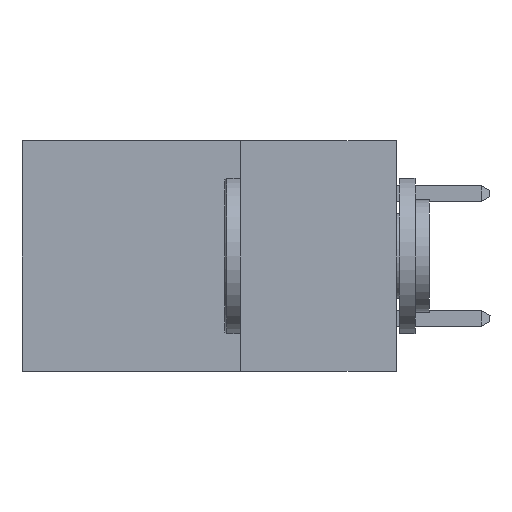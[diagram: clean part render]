
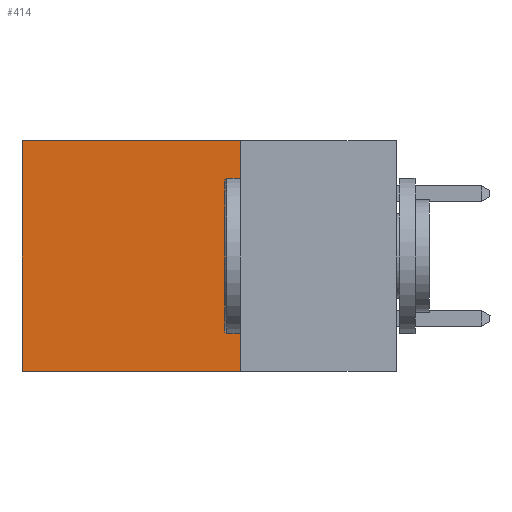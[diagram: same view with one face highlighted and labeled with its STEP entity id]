
A CAD part, left-side view. The second image highlights one B-rep face of the part: STEP entity #414.
In plain terms, the highlighted planar face has unit normal (-1, 0, 0).
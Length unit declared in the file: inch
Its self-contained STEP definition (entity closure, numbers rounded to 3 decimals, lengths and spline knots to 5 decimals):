
#123 = CARTESIAN_POINT ( 'NONE',  ( 0.2615, 0.6, -0.37 ) ) ;
#414 = ADVANCED_FACE ( 'NONE', ( #3703 ), #14101, .F. ) ;
#1155 = CARTESIAN_POINT ( 'NONE',  ( 0.2615, 0.6, 0. ) ) ;
#3271 = VECTOR ( 'NONE', #9508, 39.37008 ) ;
#3703 = FACE_OUTER_BOUND ( 'NONE', #8497, .T. ) ;
#3852 = VECTOR ( 'NONE', #13109, 39.37008 ) ;
#4131 = VERTEX_POINT ( 'NONE', #1155 ) ;
#4448 = VECTOR ( 'NONE', #7149, 39.37008 ) ;
#5177 = VERTEX_POINT ( 'NONE', #11991 ) ;
#6229 = VECTOR ( 'NONE', #7909, 39.37008 ) ;
#6248 = CARTESIAN_POINT ( 'NONE',  ( 0.2615, 0.25, -0.37 ) ) ;
#7024 = ORIENTED_EDGE ( 'NONE', *, *, #14370, .T. ) ;
#7149 = DIRECTION ( 'NONE',  ( 0., 1., 0. ) ) ;
#7431 = ORIENTED_EDGE ( 'NONE', *, *, #7670, .F. ) ;
#7547 = DIRECTION ( 'NONE',  ( 1., 0., 0. ) ) ;
#7670 = EDGE_CURVE ( 'NONE', #15599, #5177, #10167, .T. ) ;
#7909 = DIRECTION ( 'NONE',  ( 0., 0., -1. ) ) ;
#8202 = CARTESIAN_POINT ( 'NONE',  ( 0.2615, 0.25, -0.37 ) ) ;
#8461 = ORIENTED_EDGE ( 'NONE', *, *, #15417, .T. ) ;
#8497 = EDGE_LOOP ( 'NONE', ( #7024, #10496, #7431, #8461 ) ) ;
#9508 = DIRECTION ( 'NONE',  ( 0., 0., -1. ) ) ;
#10167 = LINE ( 'NONE', #8202, #3271 ) ;
#10496 = ORIENTED_EDGE ( 'NONE', *, *, #13069, .F. ) ;
#11783 = CARTESIAN_POINT ( 'NONE',  ( 0.2615, 0.25, -0.37 ) ) ;
#11800 = LINE ( 'NONE', #15019, #4448 ) ;
#11991 = CARTESIAN_POINT ( 'NONE',  ( 0.2615, 0.25, -0.37 ) ) ;
#13069 = EDGE_CURVE ( 'NONE', #5177, #16252, #14274, .T. ) ;
#13109 = DIRECTION ( 'NONE',  ( 0., 1., 0. ) ) ;
#13206 = LINE ( 'NONE', #123, #6229 ) ;
#14101 = PLANE ( 'NONE',  #14761 ) ;
#14274 = LINE ( 'NONE', #11783, #3852 ) ;
#14370 = EDGE_CURVE ( 'NONE', #4131, #16252, #13206, .T. ) ;
#14761 = AXIS2_PLACEMENT_3D ( 'NONE', #6248, #7547, #16730 ) ;
#15019 = CARTESIAN_POINT ( 'NONE',  ( 0.2615, 0.25, 0. ) ) ;
#15343 = CARTESIAN_POINT ( 'NONE',  ( 0.2615, 0.25, 0. ) ) ;
#15417 = EDGE_CURVE ( 'NONE', #15599, #4131, #11800, .T. ) ;
#15599 = VERTEX_POINT ( 'NONE', #15343 ) ;
#16099 = CARTESIAN_POINT ( 'NONE',  ( 0.2615, 0.6, -0.37 ) ) ;
#16252 = VERTEX_POINT ( 'NONE', #16099 ) ;
#16730 = DIRECTION ( 'NONE',  ( 0., 0., -1. ) ) ;
